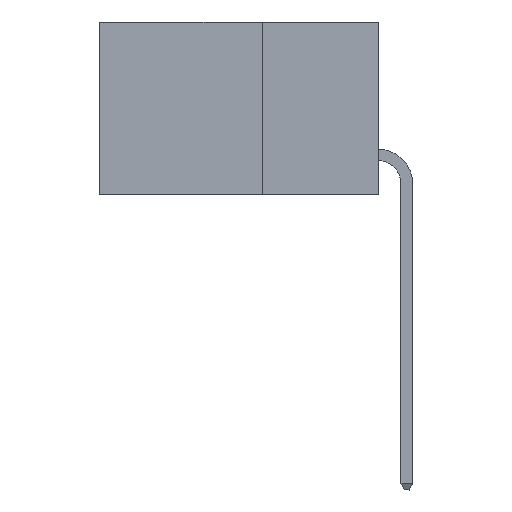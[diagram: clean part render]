
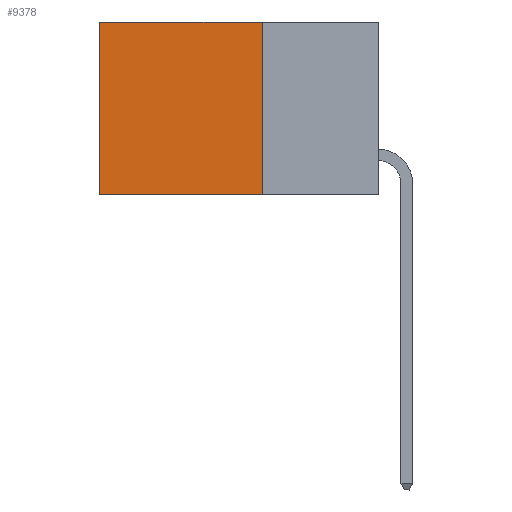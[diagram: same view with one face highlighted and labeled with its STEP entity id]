
A CAD part, left-side view. The second image highlights one B-rep face of the part: STEP entity #9378.
In plain terms, the highlighted planar face has unit normal (-1, 0, 0).
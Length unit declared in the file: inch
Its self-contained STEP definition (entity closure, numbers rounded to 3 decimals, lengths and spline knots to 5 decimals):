
#270 = VERTEX_POINT ( 'NONE', #721 ) ;
#721 = CARTESIAN_POINT ( 'NONE',  ( 0.298, 0.6, 0. ) ) ;
#883 = DIRECTION ( 'NONE',  ( 0., 0., -1. ) ) ;
#905 = EDGE_LOOP ( 'NONE', ( #14094, #8898, #6866, #4214 ) ) ;
#1057 = VECTOR ( 'NONE', #18632, 39.37008 ) ;
#1287 = DIRECTION ( 'NONE',  ( 1., 0., 0. ) ) ;
#1547 = EDGE_CURVE ( 'NONE', #14100, #270, #3145, .T. ) ;
#2165 = VECTOR ( 'NONE', #12045, 39.37008 ) ;
#2421 = LINE ( 'NONE', #16975, #4269 ) ;
#2728 = CARTESIAN_POINT ( 'NONE',  ( 0.298, 0.25, 0. ) ) ;
#2768 = DIRECTION ( 'NONE',  ( 0., 0., -1. ) ) ;
#2829 = CARTESIAN_POINT ( 'NONE',  ( 0.298, 0.25, 0. ) ) ;
#3145 = LINE ( 'NONE', #2829, #10751 ) ;
#3919 = AXIS2_PLACEMENT_3D ( 'NONE', #7152, #1287, #2768 ) ;
#4214 = ORIENTED_EDGE ( 'NONE', *, *, #1547, .T. ) ;
#4269 = VECTOR ( 'NONE', #883, 39.37008 ) ;
#4324 = DIRECTION ( 'NONE',  ( 0., 1., 0. ) ) ;
#5425 = EDGE_CURVE ( 'NONE', #14100, #11908, #2421, .T. ) ;
#5549 = PLANE ( 'NONE',  #3919 ) ;
#5950 = FACE_OUTER_BOUND ( 'NONE', #905, .T. ) ;
#5960 = EDGE_CURVE ( 'NONE', #11908, #12124, #17762, .T. ) ;
#6866 = ORIENTED_EDGE ( 'NONE', *, *, #5425, .F. ) ;
#7152 = CARTESIAN_POINT ( 'NONE',  ( 0.298, 0.25, 0. ) ) ;
#8898 = ORIENTED_EDGE ( 'NONE', *, *, #5960, .F. ) ;
#9378 = ADVANCED_FACE ( 'NONE', ( #5950 ), #5549, .F. ) ;
#9538 = CARTESIAN_POINT ( 'NONE',  ( 0.298, 0.25, -0.37 ) ) ;
#10751 = VECTOR ( 'NONE', #4324, 39.37008 ) ;
#11908 = VERTEX_POINT ( 'NONE', #9538 ) ;
#12045 = DIRECTION ( 'NONE',  ( 0., 1., 0. ) ) ;
#12124 = VERTEX_POINT ( 'NONE', #16597 ) ;
#12348 = EDGE_CURVE ( 'NONE', #270, #12124, #14140, .T. ) ;
#14094 = ORIENTED_EDGE ( 'NONE', *, *, #12348, .T. ) ;
#14100 = VERTEX_POINT ( 'NONE', #2728 ) ;
#14140 = LINE ( 'NONE', #15686, #1057 ) ;
#15686 = CARTESIAN_POINT ( 'NONE',  ( 0.298, 0.6, 0. ) ) ;
#16597 = CARTESIAN_POINT ( 'NONE',  ( 0.298, 0.6, -0.37 ) ) ;
#16975 = CARTESIAN_POINT ( 'NONE',  ( 0.298, 0.25, 0. ) ) ;
#17741 = CARTESIAN_POINT ( 'NONE',  ( 0.298, 0.25, -0.37 ) ) ;
#17762 = LINE ( 'NONE', #17741, #2165 ) ;
#18632 = DIRECTION ( 'NONE',  ( 0., 0., -1. ) ) ;
